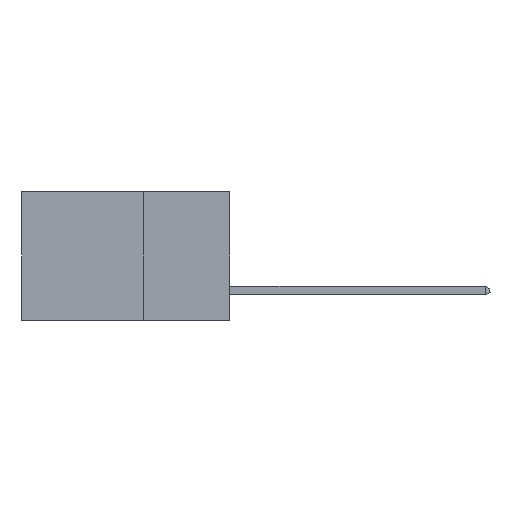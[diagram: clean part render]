
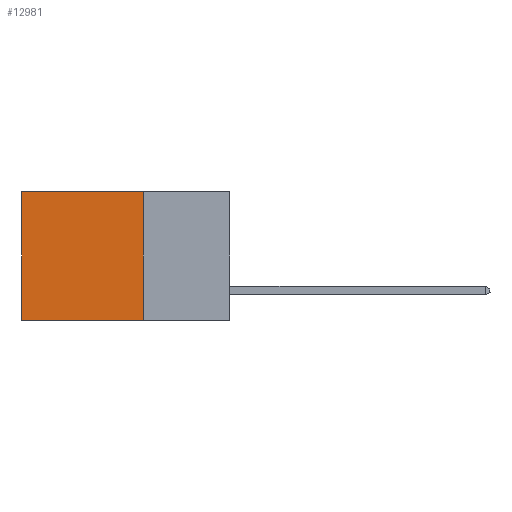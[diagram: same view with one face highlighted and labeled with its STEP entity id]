
A CAD part, left-side view. The second image highlights one B-rep face of the part: STEP entity #12981.
In plain terms, the highlighted planar face has unit normal (-1, 0, 0).
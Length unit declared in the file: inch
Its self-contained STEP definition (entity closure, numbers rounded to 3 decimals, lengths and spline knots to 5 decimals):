
#150 = VERTEX_POINT ( 'NONE', #12219 ) ;
#687 = AXIS2_PLACEMENT_3D ( 'NONE', #10990, #2631, #12951 ) ;
#1730 = DIRECTION ( 'NONE',  ( 0., 0., -1. ) ) ;
#2270 = EDGE_CURVE ( 'NONE', #150, #17615, #14392, .T. ) ;
#2631 = DIRECTION ( 'NONE',  ( 1., 0., 0. ) ) ;
#2681 = ORIENTED_EDGE ( 'NONE', *, *, #22723, .F. ) ;
#4152 = EDGE_CURVE ( 'NONE', #8494, #150, #15563, .T. ) ;
#5741 = ORIENTED_EDGE ( 'NONE', *, *, #4152, .T. ) ;
#8212 = DIRECTION ( 'NONE',  ( 0., 1., 0. ) ) ;
#8494 = VERTEX_POINT ( 'NONE', #18094 ) ;
#9569 = ORIENTED_EDGE ( 'NONE', *, *, #12304, .F. ) ;
#10099 = CARTESIAN_POINT ( 'NONE',  ( 0.298, 0.25, -0.37 ) ) ;
#10394 = EDGE_LOOP ( 'NONE', ( #10930, #2681, #9569, #5741 ) ) ;
#10930 = ORIENTED_EDGE ( 'NONE', *, *, #2270, .T. ) ;
#10990 = CARTESIAN_POINT ( 'NONE',  ( 0.298, 0.25, 0. ) ) ;
#12219 = CARTESIAN_POINT ( 'NONE',  ( 0.298, 0.6, 0. ) ) ;
#12304 = EDGE_CURVE ( 'NONE', #8494, #13679, #16027, .T. ) ;
#12951 = DIRECTION ( 'NONE',  ( 0., 0., -1. ) ) ;
#12981 = ADVANCED_FACE ( 'NONE', ( #23497 ), #15190, .F. ) ;
#13679 = VERTEX_POINT ( 'NONE', #10099 ) ;
#14392 = LINE ( 'NONE', #24336, #24724 ) ;
#15190 = PLANE ( 'NONE',  #687 ) ;
#15563 = LINE ( 'NONE', #18117, #18784 ) ;
#16027 = LINE ( 'NONE', #19063, #19308 ) ;
#16430 = CARTESIAN_POINT ( 'NONE',  ( 0.298, 0.25, -0.37 ) ) ;
#16968 = DIRECTION ( 'NONE',  ( 0., 0., -1. ) ) ;
#17615 = VERTEX_POINT ( 'NONE', #19101 ) ;
#17724 = VECTOR ( 'NONE', #8212, 39.37008 ) ;
#18094 = CARTESIAN_POINT ( 'NONE',  ( 0.298, 0.25, 0. ) ) ;
#18117 = CARTESIAN_POINT ( 'NONE',  ( 0.298, 0.25, 0. ) ) ;
#18698 = LINE ( 'NONE', #16430, #17724 ) ;
#18784 = VECTOR ( 'NONE', #20099, 39.37008 ) ;
#19063 = CARTESIAN_POINT ( 'NONE',  ( 0.298, 0.25, 0. ) ) ;
#19101 = CARTESIAN_POINT ( 'NONE',  ( 0.298, 0.6, -0.37 ) ) ;
#19308 = VECTOR ( 'NONE', #16968, 39.37008 ) ;
#20099 = DIRECTION ( 'NONE',  ( 0., 1., 0. ) ) ;
#22723 = EDGE_CURVE ( 'NONE', #13679, #17615, #18698, .T. ) ;
#23497 = FACE_OUTER_BOUND ( 'NONE', #10394, .T. ) ;
#24336 = CARTESIAN_POINT ( 'NONE',  ( 0.298, 0.6, 0. ) ) ;
#24724 = VECTOR ( 'NONE', #1730, 39.37008 ) ;
